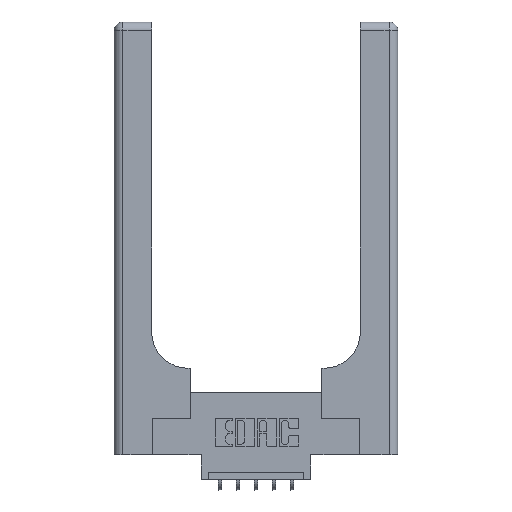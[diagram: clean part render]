
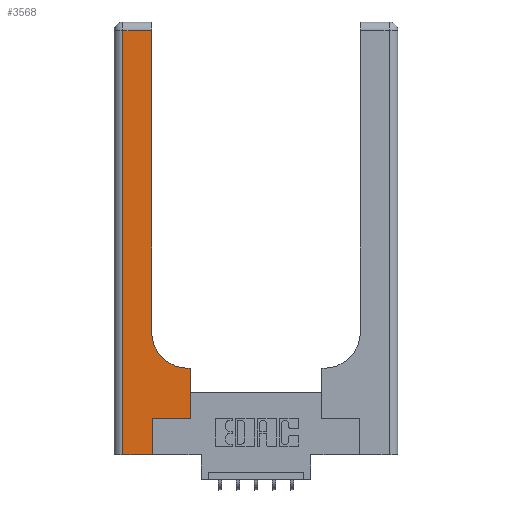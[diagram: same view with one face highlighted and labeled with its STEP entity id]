
A CAD part, top view. The second image highlights one B-rep face of the part: STEP entity #3568.
In plain terms, the highlighted planar face has unit normal (0, 0, 1).
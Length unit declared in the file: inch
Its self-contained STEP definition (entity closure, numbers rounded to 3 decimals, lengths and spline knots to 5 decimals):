
#211 = EDGE_CURVE ( 'NONE', #10633, #5270, #7142, .T. ) ;
#235 = EDGE_CURVE ( 'NONE', #9902, #1647, #10643, .T. ) ;
#256 = CARTESIAN_POINT ( 'NONE',  ( 0.26, 3., 0.37 ) ) ;
#363 = CARTESIAN_POINT ( 'NONE',  ( 0.265, 0.25, 0.37 ) ) ;
#473 = EDGE_CURVE ( 'NONE', #11650, #6396, #1871, .T. ) ;
#475 = VERTEX_POINT ( 'NONE', #4200 ) ;
#540 = ORIENTED_EDGE ( 'NONE', *, *, #6682, .T. ) ;
#1050 = DIRECTION ( 'NONE',  ( 1., 0., 0. ) ) ;
#1204 = VECTOR ( 'NONE', #10877, 39.37008 ) ;
#1218 = ORIENTED_EDGE ( 'NONE', *, *, #2653, .T. ) ;
#1275 = ORIENTED_EDGE ( 'NONE', *, *, #13303, .T. ) ;
#1647 = VERTEX_POINT ( 'NONE', #6637 ) ;
#1679 = PLANE ( 'NONE',  #10991 ) ;
#1871 = LINE ( 'NONE', #10482, #9478 ) ;
#1974 = DIRECTION ( 'NONE',  ( 0., -1., 0. ) ) ;
#2035 = CARTESIAN_POINT ( 'NONE',  ( 0.26, 0.6, 0.37 ) ) ;
#2066 = CARTESIAN_POINT ( 'NONE',  ( 0.06, 0., 0.37 ) ) ;
#2653 = EDGE_CURVE ( 'NONE', #1647, #475, #4877, .T. ) ;
#3076 = EDGE_LOOP ( 'NONE', ( #13422, #12578, #12683, #540, #12793, #1275, #10591, #12821, #1218 ) ) ;
#3568 = ADVANCED_FACE ( 'NONE', ( #5721 ), #1679, .F. ) ;
#3617 = CARTESIAN_POINT ( 'NONE',  ( 0., 3., 0.37 ) ) ;
#3748 = CARTESIAN_POINT ( 'NONE',  ( 0.528, 0.6, 0.37 ) ) ;
#3844 = VECTOR ( 'NONE', #1974, 39.37008 ) ;
#4005 = CARTESIAN_POINT ( 'NONE',  ( 0.51, 0.85, 0.37 ) ) ;
#4077 = DIRECTION ( 'NONE',  ( 0., 0., -1. ) ) ;
#4105 = VECTOR ( 'NONE', #4629, 39.37008 ) ;
#4200 = CARTESIAN_POINT ( 'NONE',  ( 0.26, 0.85, 0.37 ) ) ;
#4305 = LINE ( 'NONE', #9588, #7971 ) ;
#4323 = CARTESIAN_POINT ( 'NONE',  ( 0., 0., 0.37 ) ) ;
#4562 = CARTESIAN_POINT ( 'NONE',  ( 0.528, 0.25, 0.37 ) ) ;
#4599 = DIRECTION ( 'NONE',  ( 0., 1., 0. ) ) ;
#4629 = DIRECTION ( 'NONE',  ( 1., 0., 0. ) ) ;
#4801 = CARTESIAN_POINT ( 'NONE',  ( 0.26, 2.94, 0.37 ) ) ;
#4877 = CIRCLE ( 'NONE', #10732, 0.25 ) ;
#4922 = DIRECTION ( 'NONE',  ( 0., 0., -1. ) ) ;
#4995 = EDGE_CURVE ( 'NONE', #10742, #10633, #4305, .T. ) ;
#5126 = VECTOR ( 'NONE', #9133, 39.37008 ) ;
#5270 = VERTEX_POINT ( 'NONE', #2066 ) ;
#5418 = DIRECTION ( 'NONE',  ( -1., 0., 0. ) ) ;
#5431 = LINE ( 'NONE', #4323, #13797 ) ;
#5721 = FACE_OUTER_BOUND ( 'NONE', #3076, .T. ) ;
#5841 = CARTESIAN_POINT ( 'NONE',  ( 0.06, 2.94, 0.37 ) ) ;
#5994 = CARTESIAN_POINT ( 'NONE',  ( 0.528, 0.25, 0.37 ) ) ;
#6386 = DIRECTION ( 'NONE',  ( 1., 0., 0. ) ) ;
#6396 = VERTEX_POINT ( 'NONE', #11715 ) ;
#6400 = CARTESIAN_POINT ( 'NONE',  ( 0.06, 3., 0.37 ) ) ;
#6637 = CARTESIAN_POINT ( 'NONE',  ( 0.51, 0.6, 0.37 ) ) ;
#6682 = EDGE_CURVE ( 'NONE', #5270, #11650, #5431, .T. ) ;
#7021 = LINE ( 'NONE', #5994, #5126 ) ;
#7142 = LINE ( 'NONE', #6400, #3844 ) ;
#7389 = EDGE_CURVE ( 'NONE', #10488, #9902, #7021, .T. ) ;
#7835 = LINE ( 'NONE', #256, #10103 ) ;
#7971 = VECTOR ( 'NONE', #5418, 39.37008 ) ;
#9133 = DIRECTION ( 'NONE',  ( 0., 1., 0. ) ) ;
#9478 = VECTOR ( 'NONE', #9553, 39.37008 ) ;
#9553 = DIRECTION ( 'NONE',  ( 0., 1., 0. ) ) ;
#9588 = CARTESIAN_POINT ( 'NONE',  ( 0., 2.94, 0.37 ) ) ;
#9821 = EDGE_CURVE ( 'NONE', #475, #10742, #7835, .T. ) ;
#9902 = VERTEX_POINT ( 'NONE', #3748 ) ;
#9994 = LINE ( 'NONE', #363, #4105 ) ;
#10103 = VECTOR ( 'NONE', #4599, 39.37008 ) ;
#10156 = CARTESIAN_POINT ( 'NONE',  ( 0.265, 0., 0.37 ) ) ;
#10482 = CARTESIAN_POINT ( 'NONE',  ( 0.265, 0., 0.37 ) ) ;
#10488 = VERTEX_POINT ( 'NONE', #4562 ) ;
#10591 = ORIENTED_EDGE ( 'NONE', *, *, #7389, .T. ) ;
#10633 = VERTEX_POINT ( 'NONE', #5841 ) ;
#10643 = LINE ( 'NONE', #2035, #1204 ) ;
#10732 = AXIS2_PLACEMENT_3D ( 'NONE', #4005, #4077, #6386 ) ;
#10742 = VERTEX_POINT ( 'NONE', #4801 ) ;
#10877 = DIRECTION ( 'NONE',  ( -1., 0., 0. ) ) ;
#10991 = AXIS2_PLACEMENT_3D ( 'NONE', #3617, #4922, #13500 ) ;
#11650 = VERTEX_POINT ( 'NONE', #10156 ) ;
#11715 = CARTESIAN_POINT ( 'NONE',  ( 0.265, 0.25, 0.37 ) ) ;
#12578 = ORIENTED_EDGE ( 'NONE', *, *, #4995, .T. ) ;
#12683 = ORIENTED_EDGE ( 'NONE', *, *, #211, .T. ) ;
#12793 = ORIENTED_EDGE ( 'NONE', *, *, #473, .T. ) ;
#12821 = ORIENTED_EDGE ( 'NONE', *, *, #235, .T. ) ;
#13303 = EDGE_CURVE ( 'NONE', #6396, #10488, #9994, .T. ) ;
#13422 = ORIENTED_EDGE ( 'NONE', *, *, #9821, .T. ) ;
#13500 = DIRECTION ( 'NONE',  ( -1., 0., 0. ) ) ;
#13797 = VECTOR ( 'NONE', #1050, 39.37008 ) ;
